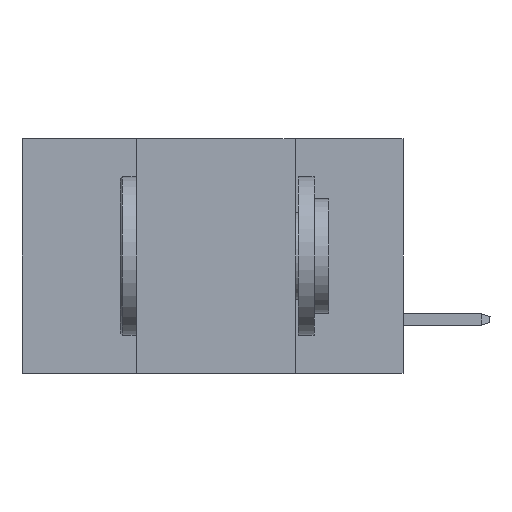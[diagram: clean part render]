
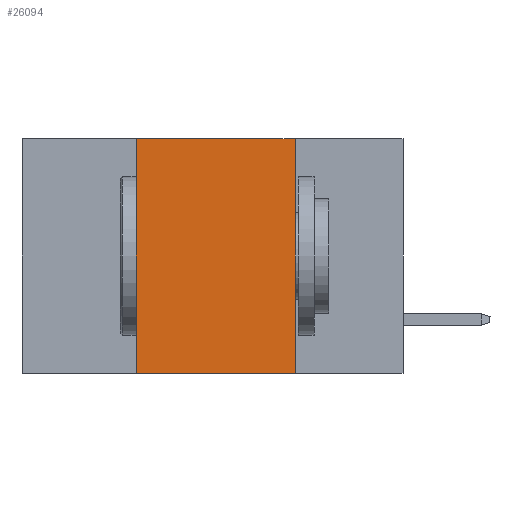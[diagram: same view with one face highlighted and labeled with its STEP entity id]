
A CAD part, left-side view. The second image highlights one B-rep face of the part: STEP entity #26094.
In plain terms, the highlighted planar face has unit normal (-1, 0, 0).
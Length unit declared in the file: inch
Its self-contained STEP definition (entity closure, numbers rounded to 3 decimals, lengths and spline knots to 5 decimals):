
#248 = LINE ( 'NONE', #14821, #18337 ) ;
#716 = CARTESIAN_POINT ( 'NONE',  ( 0., 0.17, 0. ) ) ;
#1520 = DIRECTION ( 'NONE',  ( 0., 0., 1. ) ) ;
#4404 = LINE ( 'NONE', #16803, #19476 ) ;
#4892 = VERTEX_POINT ( 'NONE', #16379 ) ;
#5093 = AXIS2_PLACEMENT_3D ( 'NONE', #23933, #23795, #13589 ) ;
#5559 = FACE_OUTER_BOUND ( 'NONE', #18288, .T. ) ;
#6199 = EDGE_CURVE ( 'NONE', #7649, #4892, #12296, .T. ) ;
#7502 = EDGE_CURVE ( 'NONE', #8930, #4892, #4404, .T. ) ;
#7649 = VERTEX_POINT ( 'NONE', #9006 ) ;
#8139 = CARTESIAN_POINT ( 'NONE',  ( 0., 0.42, 0. ) ) ;
#8415 = VECTOR ( 'NONE', #1520, 39.37008 ) ;
#8930 = VERTEX_POINT ( 'NONE', #716 ) ;
#9006 = CARTESIAN_POINT ( 'NONE',  ( 0., 0.42, -0.37 ) ) ;
#9473 = VERTEX_POINT ( 'NONE', #18404 ) ;
#9763 = PLANE ( 'NONE',  #5093 ) ;
#10513 = ORIENTED_EDGE ( 'NONE', *, *, #7502, .F. ) ;
#12296 = LINE ( 'NONE', #14882, #21281 ) ;
#13589 = DIRECTION ( 'NONE',  ( 0., 0., -1. ) ) ;
#14198 = EDGE_CURVE ( 'NONE', #9473, #8930, #248, .T. ) ;
#14821 = CARTESIAN_POINT ( 'NONE',  ( 0., 0.6, 0. ) ) ;
#14882 = CARTESIAN_POINT ( 'NONE',  ( 0., 0.6, -0.37 ) ) ;
#16365 = EDGE_CURVE ( 'NONE', #7649, #9473, #18019, .T. ) ;
#16379 = CARTESIAN_POINT ( 'NONE',  ( 0., 0.17, -0.37 ) ) ;
#16666 = DIRECTION ( 'NONE',  ( 0., 0., -1. ) ) ;
#16799 = DIRECTION ( 'NONE',  ( 0., -1., 0. ) ) ;
#16803 = CARTESIAN_POINT ( 'NONE',  ( 0., 0.17, 0. ) ) ;
#18019 = LINE ( 'NONE', #8139, #8415 ) ;
#18288 = EDGE_LOOP ( 'NONE', ( #10513, #20480, #21631, #22119 ) ) ;
#18337 = VECTOR ( 'NONE', #21072, 39.37008 ) ;
#18404 = CARTESIAN_POINT ( 'NONE',  ( 0., 0.42, 0. ) ) ;
#19476 = VECTOR ( 'NONE', #16666, 39.37008 ) ;
#20480 = ORIENTED_EDGE ( 'NONE', *, *, #14198, .F. ) ;
#21072 = DIRECTION ( 'NONE',  ( 0., -1., 0. ) ) ;
#21281 = VECTOR ( 'NONE', #16799, 39.37008 ) ;
#21631 = ORIENTED_EDGE ( 'NONE', *, *, #16365, .F. ) ;
#22119 = ORIENTED_EDGE ( 'NONE', *, *, #6199, .T. ) ;
#23795 = DIRECTION ( 'NONE',  ( 1., 0., 0. ) ) ;
#23933 = CARTESIAN_POINT ( 'NONE',  ( 0., 0.6, 0. ) ) ;
#26094 = ADVANCED_FACE ( 'NONE', ( #5559 ), #9763, .F. ) ;
